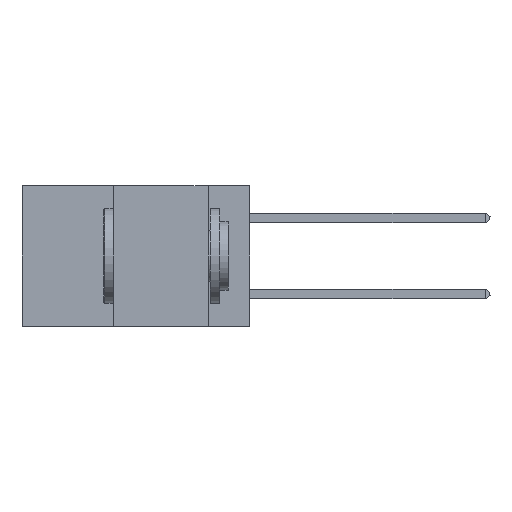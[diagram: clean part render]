
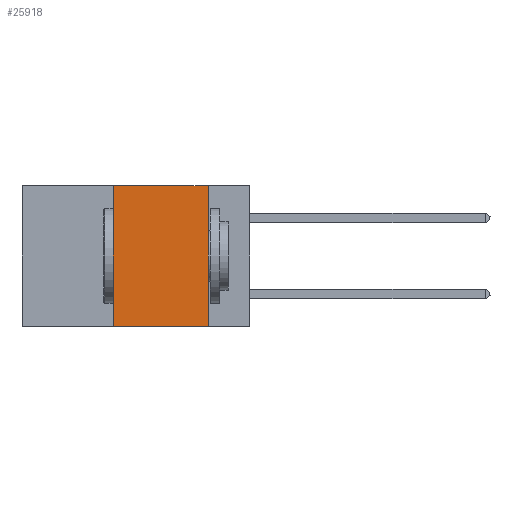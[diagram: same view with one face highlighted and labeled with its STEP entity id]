
A CAD part, left-side view. The second image highlights one B-rep face of the part: STEP entity #25918.
In plain terms, the highlighted planar face has unit normal (-1, 0, 0).
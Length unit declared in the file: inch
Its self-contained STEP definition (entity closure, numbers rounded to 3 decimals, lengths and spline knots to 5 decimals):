
#3753 = ORIENTED_EDGE ( 'NONE', *, *, #17514, .F. ) ;
#5417 = VECTOR ( 'NONE', #30588, 39.37008 ) ;
#6926 = CARTESIAN_POINT ( 'NONE',  ( 0., 0.11, -0.37 ) ) ;
#9622 = CARTESIAN_POINT ( 'NONE',  ( 0., 0.11, 0. ) ) ;
#10140 = VECTOR ( 'NONE', #29767, 39.37008 ) ;
#11927 = VERTEX_POINT ( 'NONE', #24853 ) ;
#12014 = CARTESIAN_POINT ( 'NONE',  ( 0., 0.36, 0. ) ) ;
#12089 = CARTESIAN_POINT ( 'NONE',  ( 0., 0.6, 0. ) ) ;
#12870 = CARTESIAN_POINT ( 'NONE',  ( 0., 0.6, 0. ) ) ;
#13728 = CARTESIAN_POINT ( 'NONE',  ( 0., 0.6, -0.37 ) ) ;
#13987 = FACE_OUTER_BOUND ( 'NONE', #21622, .T. ) ;
#14549 = DIRECTION ( 'NONE',  ( 0., 0., -1. ) ) ;
#16736 = CARTESIAN_POINT ( 'NONE',  ( 0., 0.36, 0. ) ) ;
#17188 = EDGE_CURVE ( 'NONE', #30925, #11927, #23022, .T. ) ;
#17324 = EDGE_CURVE ( 'NONE', #24968, #20484, #31310, .T. ) ;
#17514 = EDGE_CURVE ( 'NONE', #24968, #30925, #30922, .T. ) ;
#19259 = DIRECTION ( 'NONE',  ( 0., 0., 1. ) ) ;
#19340 = DIRECTION ( 'NONE',  ( 0., 0., -1. ) ) ;
#19584 = VECTOR ( 'NONE', #19340, 39.37008 ) ;
#20274 = ORIENTED_EDGE ( 'NONE', *, *, #17324, .T. ) ;
#20484 = VERTEX_POINT ( 'NONE', #6926 ) ;
#21622 = EDGE_LOOP ( 'NONE', ( #27439, #25356, #3753, #20274 ) ) ;
#21696 = PLANE ( 'NONE',  #28400 ) ;
#23022 = LINE ( 'NONE', #12870, #10140 ) ;
#24491 = VECTOR ( 'NONE', #19259, 39.37008 ) ;
#24853 = CARTESIAN_POINT ( 'NONE',  ( 0., 0.11, 0. ) ) ;
#24968 = VERTEX_POINT ( 'NONE', #26817 ) ;
#25356 = ORIENTED_EDGE ( 'NONE', *, *, #17188, .F. ) ;
#25918 = ADVANCED_FACE ( 'NONE', ( #13987 ), #21696, .F. ) ;
#25937 = EDGE_CURVE ( 'NONE', #11927, #20484, #26042, .T. ) ;
#26042 = LINE ( 'NONE', #9622, #19584 ) ;
#26817 = CARTESIAN_POINT ( 'NONE',  ( 0., 0.36, -0.37 ) ) ;
#27439 = ORIENTED_EDGE ( 'NONE', *, *, #25937, .F. ) ;
#28400 = AXIS2_PLACEMENT_3D ( 'NONE', #12089, #29000, #14549 ) ;
#29000 = DIRECTION ( 'NONE',  ( 1., 0., 0. ) ) ;
#29767 = DIRECTION ( 'NONE',  ( 0., -1., 0. ) ) ;
#30588 = DIRECTION ( 'NONE',  ( 0., -1., 0. ) ) ;
#30922 = LINE ( 'NONE', #12014, #24491 ) ;
#30925 = VERTEX_POINT ( 'NONE', #16736 ) ;
#31310 = LINE ( 'NONE', #13728, #5417 ) ;
